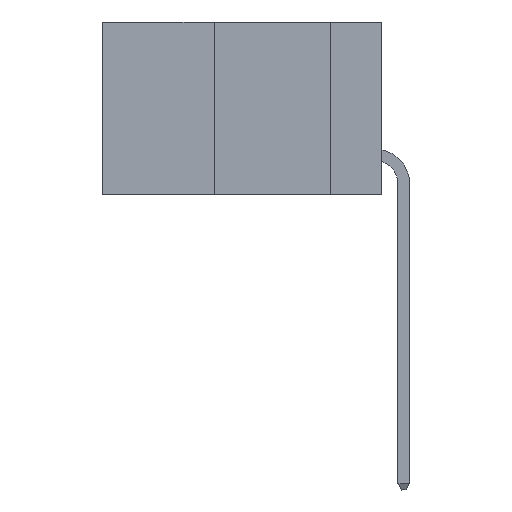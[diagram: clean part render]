
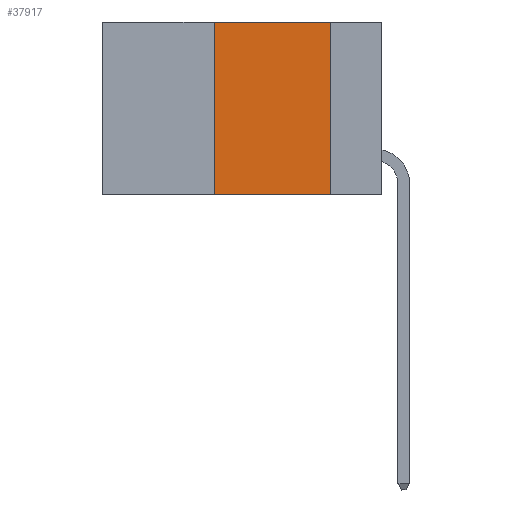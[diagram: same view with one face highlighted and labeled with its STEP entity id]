
A CAD part, left-side view. The second image highlights one B-rep face of the part: STEP entity #37917.
In plain terms, the highlighted planar face has unit normal (-1, 0, 0).
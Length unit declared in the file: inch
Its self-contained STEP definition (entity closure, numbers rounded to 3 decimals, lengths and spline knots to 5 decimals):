
#1699 = AXIS2_PLACEMENT_3D ( 'NONE', #26063, #7409, #33798 ) ;
#2953 = EDGE_LOOP ( 'NONE', ( #7214, #14656, #24526, #17307 ) ) ;
#4165 = VECTOR ( 'NONE', #19830, 39.37008 ) ;
#4749 = VECTOR ( 'NONE', #45902, 39.37008 ) ;
#4800 = EDGE_CURVE ( 'NONE', #8677, #41582, #23924, .T. ) ;
#6970 = CARTESIAN_POINT ( 'NONE',  ( 0., 0.11, 0. ) ) ;
#7214 = ORIENTED_EDGE ( 'NONE', *, *, #43433, .F. ) ;
#7409 = DIRECTION ( 'NONE',  ( 1., 0., 0. ) ) ;
#8677 = VERTEX_POINT ( 'NONE', #26219 ) ;
#9596 = LINE ( 'NONE', #11536, #4749 ) ;
#11536 = CARTESIAN_POINT ( 'NONE',  ( 0., 0.6, -0.37 ) ) ;
#14519 = PLANE ( 'NONE',  #1699 ) ;
#14656 = ORIENTED_EDGE ( 'NONE', *, *, #42852, .F. ) ;
#17307 = ORIENTED_EDGE ( 'NONE', *, *, #42984, .T. ) ;
#17381 = VECTOR ( 'NONE', #33176, 39.37008 ) ;
#18674 = CARTESIAN_POINT ( 'NONE',  ( 0., 0.11, 0. ) ) ;
#19667 = CARTESIAN_POINT ( 'NONE',  ( 0., 0.6, 0. ) ) ;
#19830 = DIRECTION ( 'NONE',  ( 0., -1., 0. ) ) ;
#21068 = VERTEX_POINT ( 'NONE', #34326 ) ;
#21301 = FACE_OUTER_BOUND ( 'NONE', #2953, .T. ) ;
#22200 = CARTESIAN_POINT ( 'NONE',  ( 0., 0.36, 0. ) ) ;
#23924 = LINE ( 'NONE', #41133, #43061 ) ;
#24526 = ORIENTED_EDGE ( 'NONE', *, *, #4800, .F. ) ;
#26063 = CARTESIAN_POINT ( 'NONE',  ( 0., 0.6, 0. ) ) ;
#26219 = CARTESIAN_POINT ( 'NONE',  ( 0., 0.36, -0.37 ) ) ;
#27506 = LINE ( 'NONE', #6970, #17381 ) ;
#28174 = LINE ( 'NONE', #19667, #4165 ) ;
#33126 = DIRECTION ( 'NONE',  ( 0., 0., 1. ) ) ;
#33176 = DIRECTION ( 'NONE',  ( 0., 0., -1. ) ) ;
#33798 = DIRECTION ( 'NONE',  ( 0., 0., -1. ) ) ;
#34326 = CARTESIAN_POINT ( 'NONE',  ( 0., 0.11, -0.37 ) ) ;
#37917 = ADVANCED_FACE ( 'NONE', ( #21301 ), #14519, .F. ) ;
#39194 = VERTEX_POINT ( 'NONE', #18674 ) ;
#41133 = CARTESIAN_POINT ( 'NONE',  ( 0., 0.36, 0. ) ) ;
#41582 = VERTEX_POINT ( 'NONE', #22200 ) ;
#42852 = EDGE_CURVE ( 'NONE', #41582, #39194, #28174, .T. ) ;
#42984 = EDGE_CURVE ( 'NONE', #8677, #21068, #9596, .T. ) ;
#43061 = VECTOR ( 'NONE', #33126, 39.37008 ) ;
#43433 = EDGE_CURVE ( 'NONE', #39194, #21068, #27506, .T. ) ;
#45902 = DIRECTION ( 'NONE',  ( 0., -1., 0. ) ) ;
